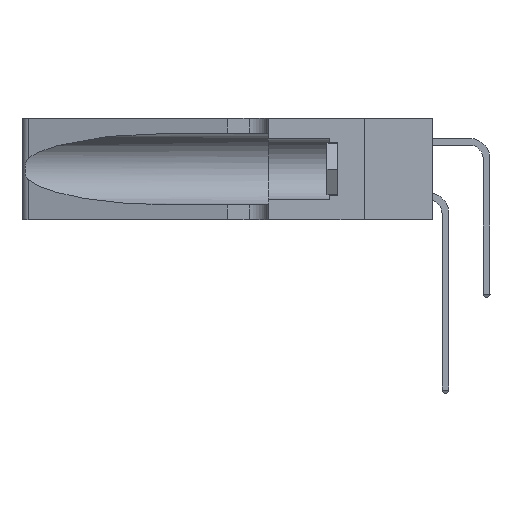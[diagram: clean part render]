
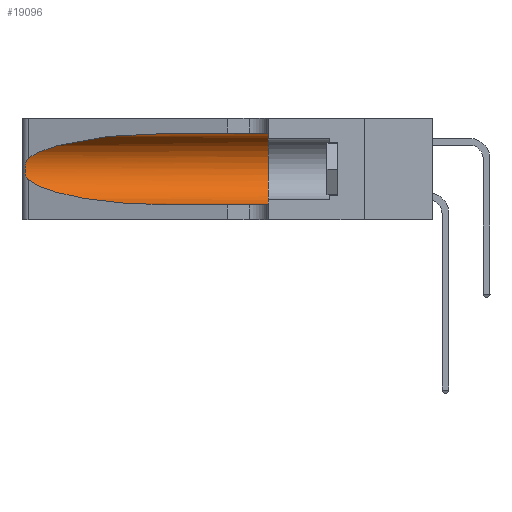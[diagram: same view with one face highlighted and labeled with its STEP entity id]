
A CAD part, left-side view. The second image highlights one B-rep face of the part: STEP entity #19096.
In plain terms, the highlighted cylindrical face has radius 3.308 mm (diameter 6.617 mm), a partial arc.
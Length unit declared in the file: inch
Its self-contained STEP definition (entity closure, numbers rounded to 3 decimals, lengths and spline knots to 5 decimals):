
#11 = CARTESIAN_POINT ( 'NONE',  ( 0.25487, 1.22718, 0.14631 ) ) ;
#1894 = EDGE_CURVE ( 'NONE', #28662, #5215, #1895, .T. ) ;
#1895 = B_SPLINE_CURVE_WITH_KNOTS ( 'NONE', 3,
 ( #2701, #27859, #36118, #22410, #5583, #25191, #8433, #27978, #11242, #30755, #14082, #33505, #16903, #11 ),
 .UNSPECIFIED., .F., .F.,
 ( 4, 2, 2, 2, 2, 2, 4 ),
 ( 0., 0.00027, 0.00053, 0.00107, 0.0016, 0.00187, 0.00214 ),
 .UNSPECIFIED. ) ;
#2054 = CARTESIAN_POINT ( 'NONE',  ( 0.1305, 0.72297, 0.31525 ) ) ;
#2289 = EDGE_LOOP ( 'NONE', ( #14470, #8387, #17417, #11195, #10593, #34879 ) ) ;
#2514 = CARTESIAN_POINT ( 'NONE',  ( 0.1305, 0.72297, 0.31525 ) ) ;
#2701 = CARTESIAN_POINT ( 'NONE',  ( 0.25487, 1.22718, 0.22369 ) ) ;
#2991 = DIRECTION ( 'NONE',  ( 0., -1., 0. ) ) ;
#3032 =( BOUNDED_CURVE ( )  B_SPLINE_CURVE ( 3, ( #2514, #33209, #8244, #27798 ),
 .UNSPECIFIED., .F., .T. ) 
 B_SPLINE_CURVE_WITH_KNOTS ( ( 4, 4 ),
 ( 1.5708, 2.84003 ),
 .UNSPECIFIED. ) 
 CURVE ( )  GEOMETRIC_REPRESENTATION_ITEM ( )  RATIONAL_B_SPLINE_CURVE ( ( 1., 0.87, 0.87, 1. ) ) 
 REPRESENTATION_ITEM ( '' )  );
#4461 = DIRECTION ( 'NONE',  ( 0., -1., 0. ) ) ;
#4565 = LINE ( 'NONE', #8420, #33372 ) ;
#5215 = VERTEX_POINT ( 'NONE', #21127 ) ;
#5583 = CARTESIAN_POINT ( 'NONE',  ( 0.25854, 1.2359, 0.20912 ) ) ;
#6075 = CARTESIAN_POINT ( 'NONE',  ( 0.1305, 0.35, 0.05475 ) ) ;
#6531 = EDGE_CURVE ( 'NONE', #22091, #9929, #13579, .T. ) ;
#8244 = CARTESIAN_POINT ( 'NONE',  ( 0.2373, 1.15595, 0.28018 ) ) ;
#8337 = CARTESIAN_POINT ( 'NONE',  ( 0.1305, 0.72297, 0.05475 ) ) ;
#8387 = ORIENTED_EDGE ( 'NONE', *, *, #1894, .T. ) ;
#8420 = CARTESIAN_POINT ( 'NONE',  ( 0.1305, 1.61858, 0.05475 ) ) ;
#8433 = CARTESIAN_POINT ( 'NONE',  ( 0.26075, 1.23896, 0.19203 ) ) ;
#8707 = CARTESIAN_POINT ( 'NONE',  ( 0.1305, 1.61858, 0.185 ) ) ;
#9024 = DIRECTION ( 'NONE',  ( 0., 1., 0. ) ) ;
#9032 = FACE_OUTER_BOUND ( 'NONE', #2289, .T. ) ;
#9929 = VERTEX_POINT ( 'NONE', #34257 ) ;
#10148 = CARTESIAN_POINT ( 'NONE',  ( 0.1305, 1.61858, 0.31525 ) ) ;
#10593 = ORIENTED_EDGE ( 'NONE', *, *, #32747, .F. ) ;
#11195 = ORIENTED_EDGE ( 'NONE', *, *, #19666, .T. ) ;
#11242 = CARTESIAN_POINT ( 'NONE',  ( 0.26017, 1.23833, 0.17102 ) ) ;
#12698 = VECTOR ( 'NONE', #4461, 39.37008 ) ;
#13579 = LINE ( 'NONE', #10148, #12698 ) ;
#14082 = CARTESIAN_POINT ( 'NONE',  ( 0.25789, 1.23486, 0.15765 ) ) ;
#14470 = ORIENTED_EDGE ( 'NONE', *, *, #23015, .T. ) ;
#16726 = CARTESIAN_POINT ( 'NONE',  ( 0.2373, 1.15595, 0.08982 ) ) ;
#16903 = CARTESIAN_POINT ( 'NONE',  ( 0.25555, 1.22993, 0.14849 ) ) ;
#17417 = ORIENTED_EDGE ( 'NONE', *, *, #36093, .T. ) ;
#17922 =( BOUNDED_CURVE ( )  B_SPLINE_CURVE ( 3, ( #33328, #16726, #36053, #19549 ),
 .UNSPECIFIED., .F., .T. ) 
 B_SPLINE_CURVE_WITH_KNOTS ( ( 4, 4 ),
 ( 3.44316, 4.71239 ),
 .UNSPECIFIED. ) 
 CURVE ( )  GEOMETRIC_REPRESENTATION_ITEM ( )  RATIONAL_B_SPLINE_CURVE ( ( 1., 0.87, 0.87, 1. ) ) 
 REPRESENTATION_ITEM ( '' )  );
#19096 = ADVANCED_FACE ( 'NONE', ( #9032 ), #23927, .F. ) ;
#19549 = CARTESIAN_POINT ( 'NONE',  ( 0.1305, 0.72297, 0.05475 ) ) ;
#19666 = EDGE_CURVE ( 'NONE', #23626, #21683, #4565, .T. ) ;
#21127 = CARTESIAN_POINT ( 'NONE',  ( 0.25487, 1.22718, 0.14631 ) ) ;
#21683 = VERTEX_POINT ( 'NONE', #6075 ) ;
#22091 = VERTEX_POINT ( 'NONE', #2054 ) ;
#22410 = CARTESIAN_POINT ( 'NONE',  ( 0.25787, 1.23484, 0.2124 ) ) ;
#23015 = EDGE_CURVE ( 'NONE', #22091, #28662, #3032, .T. ) ;
#23626 = VERTEX_POINT ( 'NONE', #8337 ) ;
#23927 = CYLINDRICAL_SURFACE ( 'NONE', #28304, 0.13025 ) ;
#25191 = CARTESIAN_POINT ( 'NONE',  ( 0.26018, 1.23835, 0.19895 ) ) ;
#25777 = CARTESIAN_POINT ( 'NONE',  ( 0.1305, 0.35, 0.185 ) ) ;
#27203 = AXIS2_PLACEMENT_3D ( 'NONE', #25777, #9024, #28558 ) ;
#27556 = CARTESIAN_POINT ( 'NONE',  ( 0.25487, 1.22718, 0.22369 ) ) ;
#27798 = CARTESIAN_POINT ( 'NONE',  ( 0.25487, 1.22718, 0.22369 ) ) ;
#27859 = CARTESIAN_POINT ( 'NONE',  ( 0.25555, 1.22994, 0.2215 ) ) ;
#27978 = CARTESIAN_POINT ( 'NONE',  ( 0.26075, 1.23896, 0.178 ) ) ;
#28090 = DIRECTION ( 'NONE',  ( 0., -1., 0. ) ) ;
#28192 = CIRCLE ( 'NONE', #27203, 0.13025 ) ;
#28253 = DIRECTION ( 'NONE',  ( 0., 0., -1. ) ) ;
#28304 = AXIS2_PLACEMENT_3D ( 'NONE', #8707, #2991, #28253 ) ;
#28558 = DIRECTION ( 'NONE',  ( 0., 0., 1. ) ) ;
#28662 = VERTEX_POINT ( 'NONE', #27556 ) ;
#30755 = CARTESIAN_POINT ( 'NONE',  ( 0.25856, 1.23593, 0.16098 ) ) ;
#32747 = EDGE_CURVE ( 'NONE', #9929, #21683, #28192, .T. ) ;
#33209 = CARTESIAN_POINT ( 'NONE',  ( 0.18966, 0.96281, 0.31525 ) ) ;
#33328 = CARTESIAN_POINT ( 'NONE',  ( 0.25487, 1.22718, 0.14631 ) ) ;
#33372 = VECTOR ( 'NONE', #28090, 39.37008 ) ;
#33505 = CARTESIAN_POINT ( 'NONE',  ( 0.25639, 1.23186, 0.15144 ) ) ;
#34257 = CARTESIAN_POINT ( 'NONE',  ( 0.1305, 0.35, 0.31525 ) ) ;
#34879 = ORIENTED_EDGE ( 'NONE', *, *, #6531, .F. ) ;
#36053 = CARTESIAN_POINT ( 'NONE',  ( 0.18966, 0.96281, 0.05475 ) ) ;
#36093 = EDGE_CURVE ( 'NONE', #5215, #23626, #17922, .T. ) ;
#36118 = CARTESIAN_POINT ( 'NONE',  ( 0.25639, 1.23184, 0.21858 ) ) ;
